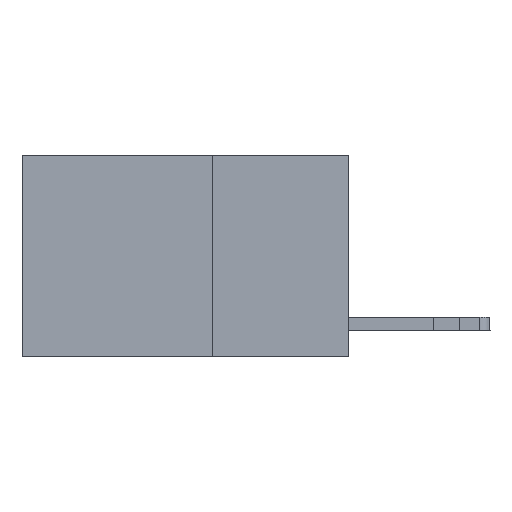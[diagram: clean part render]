
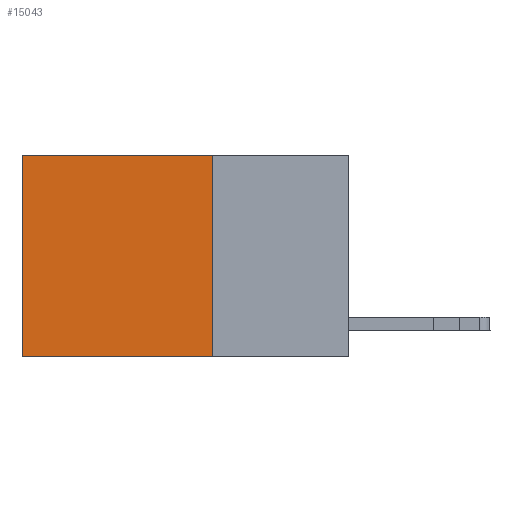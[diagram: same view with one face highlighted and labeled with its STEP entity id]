
A CAD part, left-side view. The second image highlights one B-rep face of the part: STEP entity #15043.
In plain terms, the highlighted planar face has unit normal (-1, 0, 0).
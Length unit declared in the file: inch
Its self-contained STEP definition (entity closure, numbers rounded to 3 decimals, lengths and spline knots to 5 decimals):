
#694 = ORIENTED_EDGE ( 'NONE', *, *, #11777, .T. ) ;
#1036 = AXIS2_PLACEMENT_3D ( 'NONE', #22517, #24688, #19237 ) ;
#1046 = CARTESIAN_POINT ( 'NONE',  ( 0.2625, 0.25, -0.37 ) ) ;
#1130 = VERTEX_POINT ( 'NONE', #5011 ) ;
#2371 = DIRECTION ( 'NONE',  ( 0., 0., -1. ) ) ;
#4033 = DIRECTION ( 'NONE',  ( 0., 0., -1. ) ) ;
#4102 = ORIENTED_EDGE ( 'NONE', *, *, #10453, .F. ) ;
#4651 = CARTESIAN_POINT ( 'NONE',  ( 0.2625, 0.25, 0. ) ) ;
#5011 = CARTESIAN_POINT ( 'NONE',  ( 0.2625, 0.6, -0.37 ) ) ;
#5522 = EDGE_CURVE ( 'NONE', #24052, #1130, #23331, .T. ) ;
#6068 = CARTESIAN_POINT ( 'NONE',  ( 0.2625, 0.25, 0. ) ) ;
#7676 = FACE_OUTER_BOUND ( 'NONE', #11638, .T. ) ;
#8204 = CARTESIAN_POINT ( 'NONE',  ( 0.2625, 0.25, 0. ) ) ;
#8515 = VERTEX_POINT ( 'NONE', #6068 ) ;
#9458 = VECTOR ( 'NONE', #4033, 39.37008 ) ;
#10003 = LINE ( 'NONE', #4651, #17483 ) ;
#10453 = EDGE_CURVE ( 'NONE', #8515, #17017, #18092, .T. ) ;
#11036 = ORIENTED_EDGE ( 'NONE', *, *, #5522, .T. ) ;
#11638 = EDGE_LOOP ( 'NONE', ( #11036, #12989, #4102, #694 ) ) ;
#11777 = EDGE_CURVE ( 'NONE', #8515, #24052, #10003, .T. ) ;
#12168 = CARTESIAN_POINT ( 'NONE',  ( 0.2625, 0.6, 0. ) ) ;
#12989 = ORIENTED_EDGE ( 'NONE', *, *, #15386, .F. ) ;
#15043 = ADVANCED_FACE ( 'NONE', ( #7676 ), #17215, .F. ) ;
#15386 = EDGE_CURVE ( 'NONE', #17017, #1130, #17130, .T. ) ;
#17017 = VERTEX_POINT ( 'NONE', #1046 ) ;
#17130 = LINE ( 'NONE', #24867, #22494 ) ;
#17215 = PLANE ( 'NONE',  #1036 ) ;
#17307 = VECTOR ( 'NONE', #2371, 39.37008 ) ;
#17483 = VECTOR ( 'NONE', #20228, 39.37008 ) ;
#18092 = LINE ( 'NONE', #8204, #17307 ) ;
#19237 = DIRECTION ( 'NONE',  ( 0., 0., -1. ) ) ;
#19394 = CARTESIAN_POINT ( 'NONE',  ( 0.2625, 0.6, 0. ) ) ;
#20228 = DIRECTION ( 'NONE',  ( 0., 1., 0. ) ) ;
#22494 = VECTOR ( 'NONE', #24619, 39.37008 ) ;
#22517 = CARTESIAN_POINT ( 'NONE',  ( 0.2625, 0.25, 0. ) ) ;
#23331 = LINE ( 'NONE', #19394, #9458 ) ;
#24052 = VERTEX_POINT ( 'NONE', #12168 ) ;
#24619 = DIRECTION ( 'NONE',  ( 0., 1., 0. ) ) ;
#24688 = DIRECTION ( 'NONE',  ( 1., 0., 0. ) ) ;
#24867 = CARTESIAN_POINT ( 'NONE',  ( 0.2625, 0.25, -0.37 ) ) ;
